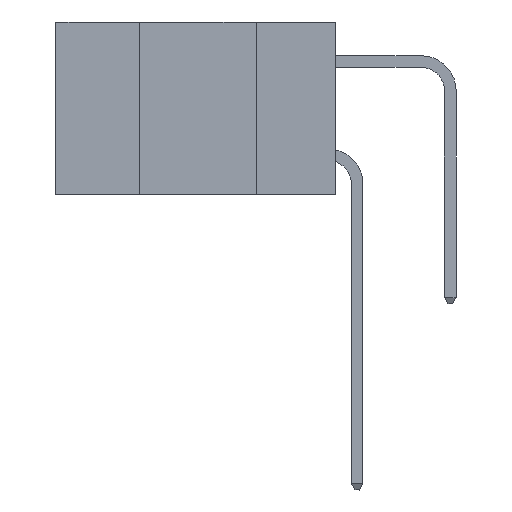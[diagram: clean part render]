
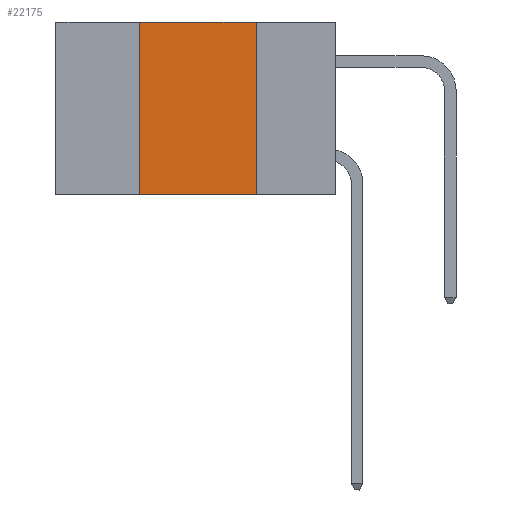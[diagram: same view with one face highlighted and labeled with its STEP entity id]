
A CAD part, left-side view. The second image highlights one B-rep face of the part: STEP entity #22175.
In plain terms, the highlighted planar face has unit normal (-1, 0, 0).
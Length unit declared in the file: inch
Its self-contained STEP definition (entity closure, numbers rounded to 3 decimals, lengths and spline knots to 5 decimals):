
#1227 = EDGE_CURVE ( 'NONE', #29496, #41337, #5046, .T. ) ;
#1513 = EDGE_CURVE ( 'NONE', #29394, #29496, #30069, .T. ) ;
#3193 = EDGE_CURVE ( 'NONE', #22076, #29394, #27027, .T. ) ;
#4528 = EDGE_CURVE ( 'NONE', #22076, #41337, #30455, .T. ) ;
#5046 = LINE ( 'NONE', #27970, #9149 ) ;
#6223 = ORIENTED_EDGE ( 'NONE', *, *, #3193, .F. ) ;
#7361 = DIRECTION ( 'NONE',  ( 0., -1., 0. ) ) ;
#7762 = CARTESIAN_POINT ( 'NONE',  ( 0., 0.6, -0.37 ) ) ;
#8306 = DIRECTION ( 'NONE',  ( 0., 0., -1. ) ) ;
#9149 = VECTOR ( 'NONE', #21542, 39.37008 ) ;
#10511 = PLANE ( 'NONE',  #16195 ) ;
#16195 = AXIS2_PLACEMENT_3D ( 'NONE', #23568, #34017, #8306 ) ;
#17794 = CARTESIAN_POINT ( 'NONE',  ( 0., 0.42, 0. ) ) ;
#17873 = EDGE_LOOP ( 'NONE', ( #21669, #21571, #6223, #39894 ) ) ;
#18433 = VECTOR ( 'NONE', #7361, 39.37008 ) ;
#20176 = DIRECTION ( 'NONE',  ( 0., 0., 1. ) ) ;
#20496 = CARTESIAN_POINT ( 'NONE',  ( 0., 0.17, 0. ) ) ;
#21542 = DIRECTION ( 'NONE',  ( 0., 0., -1. ) ) ;
#21571 = ORIENTED_EDGE ( 'NONE', *, *, #1513, .F. ) ;
#21669 = ORIENTED_EDGE ( 'NONE', *, *, #1227, .F. ) ;
#22076 = VERTEX_POINT ( 'NONE', #30786 ) ;
#22175 = ADVANCED_FACE ( 'NONE', ( #39851 ), #10511, .F. ) ;
#23568 = CARTESIAN_POINT ( 'NONE',  ( 0., 0.6, 0. ) ) ;
#27027 = LINE ( 'NONE', #17794, #37972 ) ;
#27462 = DIRECTION ( 'NONE',  ( 0., -1., 0. ) ) ;
#27970 = CARTESIAN_POINT ( 'NONE',  ( 0., 0.17, 0. ) ) ;
#29394 = VERTEX_POINT ( 'NONE', #39789 ) ;
#29496 = VERTEX_POINT ( 'NONE', #20496 ) ;
#30069 = LINE ( 'NONE', #30699, #18433 ) ;
#30455 = LINE ( 'NONE', #7762, #30525 ) ;
#30525 = VECTOR ( 'NONE', #27462, 39.37008 ) ;
#30699 = CARTESIAN_POINT ( 'NONE',  ( 0., 0.6, 0. ) ) ;
#30786 = CARTESIAN_POINT ( 'NONE',  ( 0., 0.42, -0.37 ) ) ;
#33917 = CARTESIAN_POINT ( 'NONE',  ( 0., 0.17, -0.37 ) ) ;
#34017 = DIRECTION ( 'NONE',  ( 1., 0., 0. ) ) ;
#37972 = VECTOR ( 'NONE', #20176, 39.37008 ) ;
#39789 = CARTESIAN_POINT ( 'NONE',  ( 0., 0.42, 0. ) ) ;
#39851 = FACE_OUTER_BOUND ( 'NONE', #17873, .T. ) ;
#39894 = ORIENTED_EDGE ( 'NONE', *, *, #4528, .T. ) ;
#41337 = VERTEX_POINT ( 'NONE', #33917 ) ;
